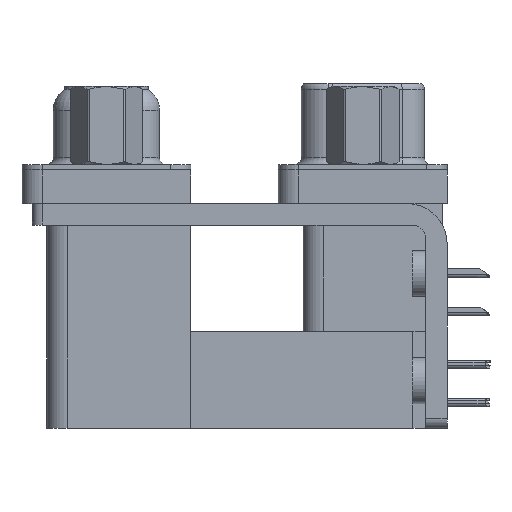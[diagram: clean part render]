
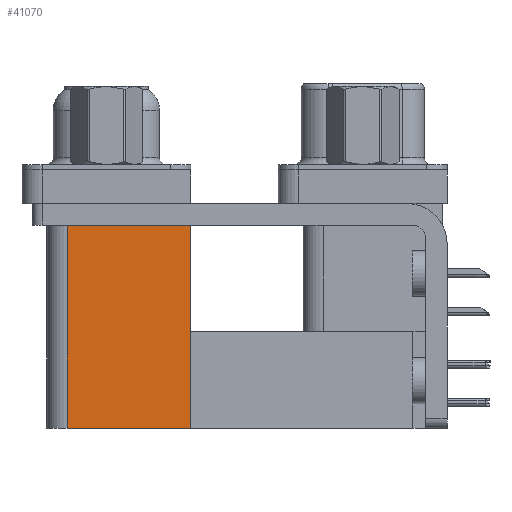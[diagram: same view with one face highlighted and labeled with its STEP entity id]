
A CAD part, left-side view. The second image highlights one B-rep face of the part: STEP entity #41070.
In plain terms, the highlighted planar face has unit normal (-1, 0, 0).
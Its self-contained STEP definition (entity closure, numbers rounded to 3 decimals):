
#358 = CARTESIAN_POINT ( 'NONE',  ( 3.765, 12.775, -19.2 ) ) ;
#872 = LINE ( 'NONE', #358, #9412 ) ;
#3640 = EDGE_CURVE ( 'NONE', #45792, #35011, #47198, .T. ) ;
#3971 = AXIS2_PLACEMENT_3D ( 'NONE', #10842, #14746, #30570 ) ;
#4663 = VERTEX_POINT ( 'NONE', #6760 ) ;
#5545 = VECTOR ( 'NONE', #6274, 1000. ) ;
#5598 = CARTESIAN_POINT ( 'NONE',  ( 3.765, 12.775, -2.5 ) ) ;
#5782 = LINE ( 'NONE', #48871, #5545 ) ;
#6274 = DIRECTION ( 'NONE',  ( 0., 0., 1. ) ) ;
#6284 = CARTESIAN_POINT ( 'NONE',  ( 3.765, 21.975, -2.5 ) ) ;
#6760 = CARTESIAN_POINT ( 'NONE',  ( 3.765, 21.975, -19.2 ) ) ;
#7148 = CARTESIAN_POINT ( 'NONE',  ( 3.765, 12.775, -19.2 ) ) ;
#9412 = VECTOR ( 'NONE', #23482, 1000. ) ;
#10842 = CARTESIAN_POINT ( 'NONE',  ( 3.765, 12.775, -19.2 ) ) ;
#14226 = PLANE ( 'NONE',  #3971 ) ;
#14746 = DIRECTION ( 'NONE',  ( 1., 0., 0. ) ) ;
#18513 = ORIENTED_EDGE ( 'NONE', *, *, #29245, .F. ) ;
#20564 = CARTESIAN_POINT ( 'NONE',  ( 3.765, 12.775, -19.2 ) ) ;
#20727 = EDGE_CURVE ( 'NONE', #4663, #35011, #5782, .T. ) ;
#22651 = ORIENTED_EDGE ( 'NONE', *, *, #49178, .T. ) ;
#23482 = DIRECTION ( 'NONE',  ( 0., 0., 1. ) ) ;
#28385 = EDGE_LOOP ( 'NONE', ( #37692, #35766, #18513, #22651 ) ) ;
#29245 = EDGE_CURVE ( 'NONE', #35168, #4663, #34404, .T. ) ;
#30570 = DIRECTION ( 'NONE',  ( 0., 1., 0. ) ) ;
#30768 = DIRECTION ( 'NONE',  ( 0., 1., 0. ) ) ;
#31084 = VECTOR ( 'NONE', #30768, 1000. ) ;
#32170 = VECTOR ( 'NONE', #40146, 1000. ) ;
#34404 = LINE ( 'NONE', #7148, #31084 ) ;
#34649 = CARTESIAN_POINT ( 'NONE',  ( 3.765, 12.775, -2.5 ) ) ;
#35011 = VERTEX_POINT ( 'NONE', #6284 ) ;
#35168 = VERTEX_POINT ( 'NONE', #20564 ) ;
#35766 = ORIENTED_EDGE ( 'NONE', *, *, #20727, .F. ) ;
#37692 = ORIENTED_EDGE ( 'NONE', *, *, #3640, .T. ) ;
#37853 = FACE_OUTER_BOUND ( 'NONE', #28385, .T. ) ;
#40146 = DIRECTION ( 'NONE',  ( 0., 1., 0. ) ) ;
#41070 = ADVANCED_FACE ( 'NONE', ( #37853 ), #14226, .F. ) ;
#45792 = VERTEX_POINT ( 'NONE', #5598 ) ;
#47198 = LINE ( 'NONE', #34649, #32170 ) ;
#48871 = CARTESIAN_POINT ( 'NONE',  ( 3.765, 21.975, -19.2 ) ) ;
#49178 = EDGE_CURVE ( 'NONE', #35168, #45792, #872, .T. ) ;
